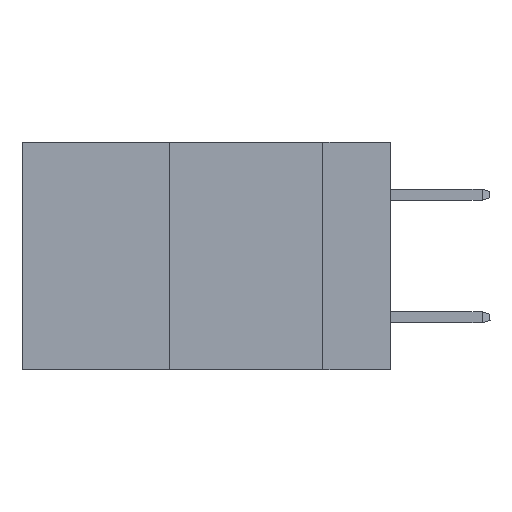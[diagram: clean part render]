
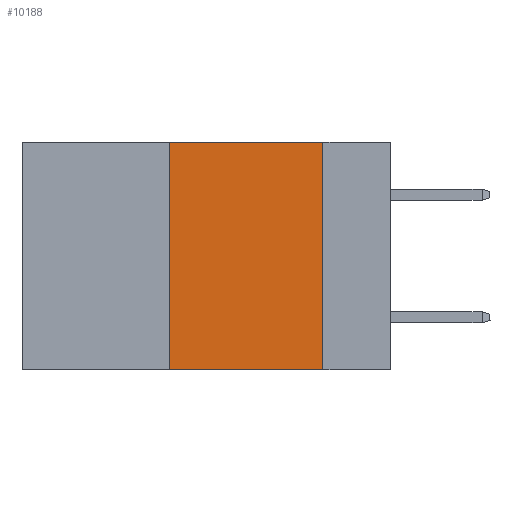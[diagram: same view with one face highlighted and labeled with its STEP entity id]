
A CAD part, left-side view. The second image highlights one B-rep face of the part: STEP entity #10188.
In plain terms, the highlighted planar face has unit normal (-1, 0, 0).
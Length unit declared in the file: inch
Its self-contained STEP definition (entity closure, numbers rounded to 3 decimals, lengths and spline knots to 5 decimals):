
#602 = CARTESIAN_POINT ( 'NONE',  ( 0., 0.11, 0. ) ) ;
#1069 = DIRECTION ( 'NONE',  ( 1., 0., 0. ) ) ;
#1214 = CARTESIAN_POINT ( 'NONE',  ( 0., 0.11, -0.37 ) ) ;
#1274 = VECTOR ( 'NONE', #11154, 39.37008 ) ;
#1776 = VECTOR ( 'NONE', #5299, 39.37008 ) ;
#2071 = CARTESIAN_POINT ( 'NONE',  ( 0., 0.11, 0. ) ) ;
#2340 = LINE ( 'NONE', #7249, #1776 ) ;
#3102 = CARTESIAN_POINT ( 'NONE',  ( 0., 0.6, 0. ) ) ;
#3190 = EDGE_CURVE ( 'NONE', #8117, #10793, #7335, .T. ) ;
#3371 = CARTESIAN_POINT ( 'NONE',  ( 0., 0.36, 0. ) ) ;
#3476 = DIRECTION ( 'NONE',  ( 0., -1., 0. ) ) ;
#3478 = ORIENTED_EDGE ( 'NONE', *, *, #4624, .F. ) ;
#4030 = VERTEX_POINT ( 'NONE', #1214 ) ;
#4624 = EDGE_CURVE ( 'NONE', #10793, #4030, #5521, .T. ) ;
#4831 = VECTOR ( 'NONE', #3476, 39.37008 ) ;
#5299 = DIRECTION ( 'NONE',  ( 0., 0., 1. ) ) ;
#5384 = CARTESIAN_POINT ( 'NONE',  ( 0., 0.6, 0. ) ) ;
#5521 = LINE ( 'NONE', #602, #12077 ) ;
#6313 = FACE_OUTER_BOUND ( 'NONE', #9058, .T. ) ;
#6378 = LINE ( 'NONE', #12342, #4831 ) ;
#6822 = EDGE_CURVE ( 'NONE', #11111, #4030, #6378, .T. ) ;
#6844 = ORIENTED_EDGE ( 'NONE', *, *, #3190, .F. ) ;
#7113 = CARTESIAN_POINT ( 'NONE',  ( 0., 0.36, -0.37 ) ) ;
#7249 = CARTESIAN_POINT ( 'NONE',  ( 0., 0.36, 0. ) ) ;
#7335 = LINE ( 'NONE', #5384, #1274 ) ;
#7867 = AXIS2_PLACEMENT_3D ( 'NONE', #3102, #1069, #12087 ) ;
#8061 = ORIENTED_EDGE ( 'NONE', *, *, #6822, .T. ) ;
#8117 = VERTEX_POINT ( 'NONE', #3371 ) ;
#8968 = PLANE ( 'NONE',  #7867 ) ;
#9058 = EDGE_LOOP ( 'NONE', ( #3478, #6844, #11493, #8061 ) ) ;
#9407 = EDGE_CURVE ( 'NONE', #11111, #8117, #2340, .T. ) ;
#10188 = ADVANCED_FACE ( 'NONE', ( #6313 ), #8968, .F. ) ;
#10644 = DIRECTION ( 'NONE',  ( 0., 0., -1. ) ) ;
#10793 = VERTEX_POINT ( 'NONE', #2071 ) ;
#11111 = VERTEX_POINT ( 'NONE', #7113 ) ;
#11154 = DIRECTION ( 'NONE',  ( 0., -1., 0. ) ) ;
#11493 = ORIENTED_EDGE ( 'NONE', *, *, #9407, .F. ) ;
#12077 = VECTOR ( 'NONE', #10644, 39.37008 ) ;
#12087 = DIRECTION ( 'NONE',  ( 0., 0., -1. ) ) ;
#12342 = CARTESIAN_POINT ( 'NONE',  ( 0., 0.6, -0.37 ) ) ;
